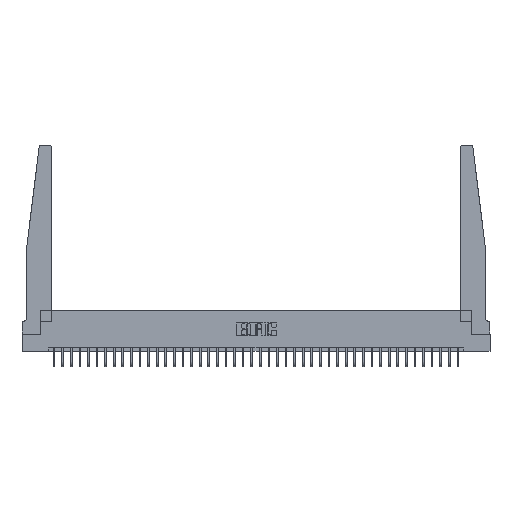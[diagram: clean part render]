
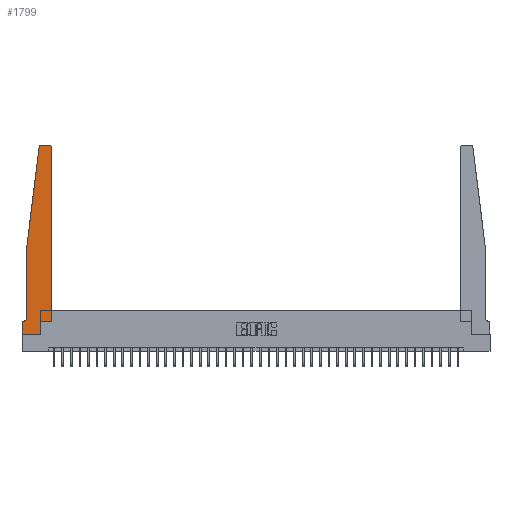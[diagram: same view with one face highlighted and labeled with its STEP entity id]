
A CAD part, top view. The second image highlights one B-rep face of the part: STEP entity #1799.
In plain terms, the highlighted planar face has unit normal (0, 0, 1).
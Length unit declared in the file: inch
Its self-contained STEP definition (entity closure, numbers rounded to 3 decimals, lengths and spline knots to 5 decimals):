
#519 = CARTESIAN_POINT ( 'NONE',  ( 0.395, 2.75, 0.37 ) ) ;
#890 = LINE ( 'NONE', #34177, #21056 ) ;
#1436 = CARTESIAN_POINT ( 'NONE',  ( 0.2605, 0.18, 0.37 ) ) ;
#1799 = ADVANCED_FACE ( 'NONE', ( #7792 ), #4140, .T. ) ;
#1842 = CARTESIAN_POINT ( 'NONE',  ( 0.065, 1.25, 0.37 ) ) ;
#1875 = CARTESIAN_POINT ( 'NONE',  ( 0., 0., 0.37 ) ) ;
#1978 = LINE ( 'NONE', #3955, #15394 ) ;
#2409 = VECTOR ( 'NONE', #27600, 39.37008 ) ;
#2587 = DIRECTION ( 'NONE',  ( 0., 0., -1. ) ) ;
#2935 = EDGE_CURVE ( 'NONE', #27327, #13505, #21213, .T. ) ;
#3124 = DIRECTION ( 'NONE',  ( 0., 1., 0. ) ) ;
#3436 = DIRECTION ( 'NONE',  ( 0., 0., 1. ) ) ;
#3955 = CARTESIAN_POINT ( 'NONE',  ( 0., 0., 0.37 ) ) ;
#4140 = PLANE ( 'NONE',  #9435 ) ;
#4278 = DIRECTION ( 'NONE',  ( 1., 0., 0. ) ) ;
#6438 = VECTOR ( 'NONE', #26404, 39.37008 ) ;
#7792 = FACE_OUTER_BOUND ( 'NONE', #34512, .T. ) ;
#8037 = LINE ( 'NONE', #17250, #10724 ) ;
#8055 = EDGE_CURVE ( 'NONE', #29346, #29652, #32043, .T. ) ;
#8503 = CARTESIAN_POINT ( 'NONE',  ( 0.2605, 0.18, 0.37 ) ) ;
#8577 = DIRECTION ( 'NONE',  ( -1., 0., 0. ) ) ;
#8687 = CARTESIAN_POINT ( 'NONE',  ( 0.27653, 2.72, 0.37 ) ) ;
#8734 = EDGE_CURVE ( 'NONE', #21795, #11133, #13976, .T. ) ;
#9435 = AXIS2_PLACEMENT_3D ( 'NONE', #12739, #17854, #4278 ) ;
#10036 = CIRCLE ( 'NONE', #23591, 0.05 ) ;
#10122 = AXIS2_PLACEMENT_3D ( 'NONE', #21351, #35697, #15567 ) ;
#10549 = EDGE_CURVE ( 'NONE', #15862, #21795, #29674, .T. ) ;
#10724 = VECTOR ( 'NONE', #11614, 39.37008 ) ;
#11133 = VERTEX_POINT ( 'NONE', #24165 ) ;
#11169 = ORIENTED_EDGE ( 'NONE', *, *, #31756, .T. ) ;
#11614 = DIRECTION ( 'NONE',  ( 0., 1., 0. ) ) ;
#12101 = CARTESIAN_POINT ( 'NONE',  ( 0.425, 0.18, 0.37 ) ) ;
#12433 = ORIENTED_EDGE ( 'NONE', *, *, #20754, .T. ) ;
#12739 = CARTESIAN_POINT ( 'NONE',  ( 0., 0.1875, 0.37 ) ) ;
#13001 = CARTESIAN_POINT ( 'NONE',  ( 0.065, 0.1875, 0.37 ) ) ;
#13258 = CARTESIAN_POINT ( 'NONE',  ( 0., 0.1875, 0.37 ) ) ;
#13505 = VERTEX_POINT ( 'NONE', #1436 ) ;
#13691 = CARTESIAN_POINT ( 'NONE',  ( 0.015, 0.2375, 0.37 ) ) ;
#13976 = LINE ( 'NONE', #16092, #23469 ) ;
#14211 = CIRCLE ( 'NONE', #19307, 0.03 ) ;
#14228 = VERTEX_POINT ( 'NONE', #1875 ) ;
#14431 = ORIENTED_EDGE ( 'NONE', *, *, #25036, .T. ) ;
#14506 = ORIENTED_EDGE ( 'NONE', *, *, #19447, .T. ) ;
#14591 = LINE ( 'NONE', #1842, #32550 ) ;
#15394 = VECTOR ( 'NONE', #17922, 39.37008 ) ;
#15567 = DIRECTION ( 'NONE',  ( 1., 0., 0. ) ) ;
#15585 = CARTESIAN_POINT ( 'NONE',  ( 0.065, 1.25, 0.37 ) ) ;
#15862 = VERTEX_POINT ( 'NONE', #15877 ) ;
#15877 = CARTESIAN_POINT ( 'NONE',  ( 0.425, 2.72, 0.37 ) ) ;
#16092 = CARTESIAN_POINT ( 'NONE',  ( 0.25, 2.75, 0.37 ) ) ;
#16444 = EDGE_CURVE ( 'NONE', #14228, #27327, #1978, .T. ) ;
#17250 = CARTESIAN_POINT ( 'NONE',  ( 0.425, 0.18, 0.37 ) ) ;
#17386 = EDGE_CURVE ( 'NONE', #32268, #33769, #25237, .T. ) ;
#17545 = VERTEX_POINT ( 'NONE', #24903 ) ;
#17854 = DIRECTION ( 'NONE',  ( 0., 0., 1. ) ) ;
#17922 = DIRECTION ( 'NONE',  ( 1., 0., 0. ) ) ;
#18022 = CARTESIAN_POINT ( 'NONE',  ( 0.015, 0.1875, 0.37 ) ) ;
#18986 = ORIENTED_EDGE ( 'NONE', *, *, #2935, .T. ) ;
#19307 = AXIS2_PLACEMENT_3D ( 'NONE', #8687, #3436, #31533 ) ;
#19447 = EDGE_CURVE ( 'NONE', #17545, #32268, #14591, .T. ) ;
#19466 = ORIENTED_EDGE ( 'NONE', *, *, #8055, .T. ) ;
#19879 = ORIENTED_EDGE ( 'NONE', *, *, #31834, .T. ) ;
#20754 = EDGE_CURVE ( 'NONE', #33769, #29346, #10036, .T. ) ;
#20933 = EDGE_CURVE ( 'NONE', #29652, #14228, #23524, .T. ) ;
#21056 = VECTOR ( 'NONE', #23329, 39.37008 ) ;
#21213 = LINE ( 'NONE', #8503, #34709 ) ;
#21351 = CARTESIAN_POINT ( 'NONE',  ( 0.395, 2.72, 0.37 ) ) ;
#21496 = DIRECTION ( 'NONE',  ( 0., -1., 0. ) ) ;
#21795 = VERTEX_POINT ( 'NONE', #519 ) ;
#21888 = DIRECTION ( 'NONE',  ( -1., 0., 0. ) ) ;
#22101 = ORIENTED_EDGE ( 'NONE', *, *, #20933, .T. ) ;
#23009 = VECTOR ( 'NONE', #21496, 39.37008 ) ;
#23329 = DIRECTION ( 'NONE',  ( 1., 0., 0. ) ) ;
#23469 = VECTOR ( 'NONE', #21888, 39.37008 ) ;
#23524 = LINE ( 'NONE', #28931, #6438 ) ;
#23591 = AXIS2_PLACEMENT_3D ( 'NONE', #13691, #2587, #8577 ) ;
#24165 = CARTESIAN_POINT ( 'NONE',  ( 0.27653, 2.75, 0.37 ) ) ;
#24623 = ORIENTED_EDGE ( 'NONE', *, *, #10549, .T. ) ;
#24903 = CARTESIAN_POINT ( 'NONE',  ( 0.24675, 2.72367, 0.37 ) ) ;
#24944 = DIRECTION ( 'NONE',  ( -0.122, -0.992, 0. ) ) ;
#25036 = EDGE_CURVE ( 'NONE', #11133, #17545, #14211, .T. ) ;
#25237 = LINE ( 'NONE', #15585, #23009 ) ;
#25258 = CARTESIAN_POINT ( 'NONE',  ( 0.065, 1.25, 0.37 ) ) ;
#26234 = ORIENTED_EDGE ( 'NONE', *, *, #17386, .T. ) ;
#26404 = DIRECTION ( 'NONE',  ( 0., -1., 0. ) ) ;
#27327 = VERTEX_POINT ( 'NONE', #36133 ) ;
#27600 = DIRECTION ( 'NONE',  ( -1., 0., 0. ) ) ;
#28931 = CARTESIAN_POINT ( 'NONE',  ( 0., 0., 0.37 ) ) ;
#29176 = CARTESIAN_POINT ( 'NONE',  ( 0.065, 0.2375, 0.37 ) ) ;
#29346 = VERTEX_POINT ( 'NONE', #18022 ) ;
#29652 = VERTEX_POINT ( 'NONE', #13258 ) ;
#29674 = CIRCLE ( 'NONE', #10122, 0.03 ) ;
#30138 = VERTEX_POINT ( 'NONE', #12101 ) ;
#31076 = ORIENTED_EDGE ( 'NONE', *, *, #8734, .T. ) ;
#31533 = DIRECTION ( 'NONE',  ( 1., 0., 0. ) ) ;
#31756 = EDGE_CURVE ( 'NONE', #13505, #30138, #890, .T. ) ;
#31834 = EDGE_CURVE ( 'NONE', #30138, #15862, #8037, .T. ) ;
#32043 = LINE ( 'NONE', #13001, #2409 ) ;
#32268 = VERTEX_POINT ( 'NONE', #25258 ) ;
#32550 = VECTOR ( 'NONE', #24944, 39.37008 ) ;
#33769 = VERTEX_POINT ( 'NONE', #29176 ) ;
#34177 = CARTESIAN_POINT ( 'NONE',  ( 0.425, 0.18, 0.37 ) ) ;
#34270 = ORIENTED_EDGE ( 'NONE', *, *, #16444, .T. ) ;
#34512 = EDGE_LOOP ( 'NONE', ( #31076, #14431, #14506, #26234, #12433, #19466, #22101, #34270, #18986, #11169, #19879, #24623 ) ) ;
#34709 = VECTOR ( 'NONE', #3124, 39.37008 ) ;
#35697 = DIRECTION ( 'NONE',  ( 0., 0., 1. ) ) ;
#36133 = CARTESIAN_POINT ( 'NONE',  ( 0.2605, 0., 0.37 ) ) ;
